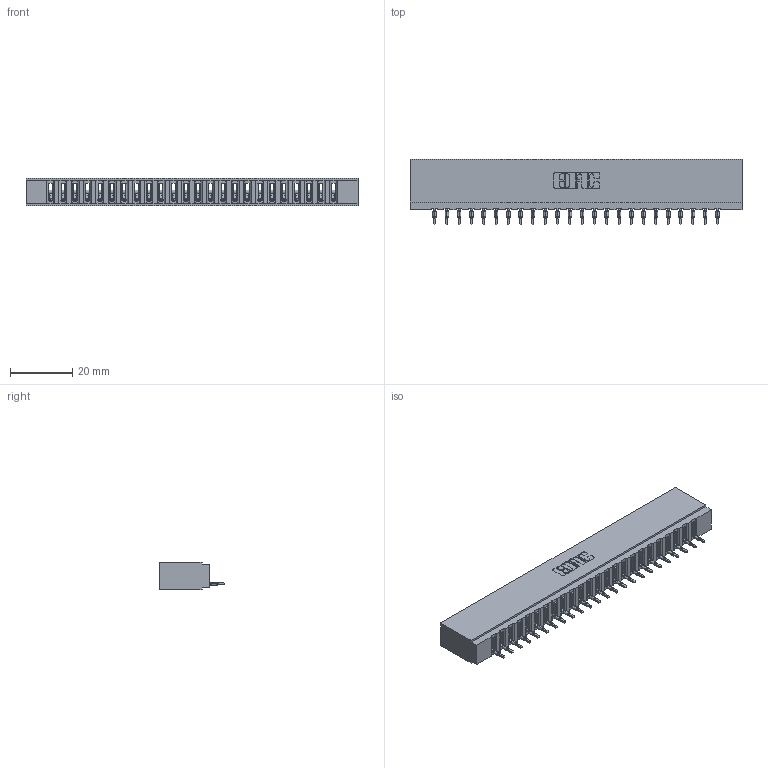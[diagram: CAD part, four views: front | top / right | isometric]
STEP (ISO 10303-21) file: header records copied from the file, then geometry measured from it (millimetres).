
FILE_DESCRIPTION (( 'STEP AP203' ), '1' );
FILE_NAME ('737-024-525-101.STEP', '2020-09-10T21:52:55', ( '' ), ( '' ), 'SwSTEP 2.0', 'SolidWorks 2020', '' );
FILE_SCHEMA (( 'CONFIG_CONTROL_DESIGN' ));
Length unit declared in the file: inch
Products named in the file (3): 745-292-001_525; 737-024-525-101; 737 Part_Insulator Option - 01
Assembly tree (25 placements, depth 2):
  737-024-525-101
    737 Part_Insulator Option - 01
    745-292-001_525  x24
Bounding box: 106.93 x 21.22 x 8.89 mm (x, y, z)
Volume: 10441.8 mm3; surface area: 13631.6 mm2
Topology: 25 solids, 25 shells, 2806 faces, 7719 edges, 4874 vertices
Faces by surface type: plane 1686, cylinder 496, bspline 480, torus 144
Entity records: 42859 total; most frequent: CARTESIAN_POINT 8057, ORIENTED_EDGE 7480, DIRECTION 6496, EDGE_CURVE 3740, LINE 3414, VECTOR 3414, VERTEX_POINT 2390, AXIS2_PLACEMENT_3D 1541
